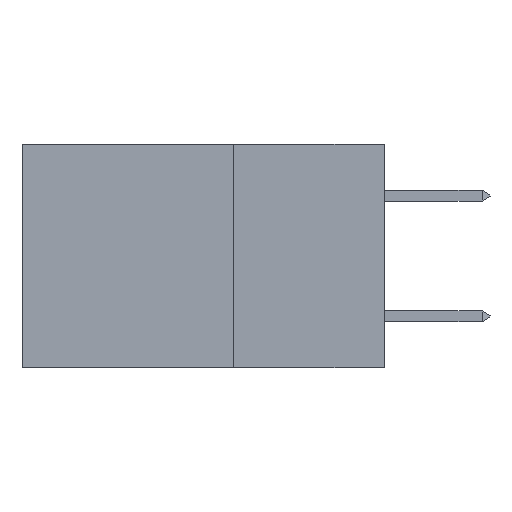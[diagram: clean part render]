
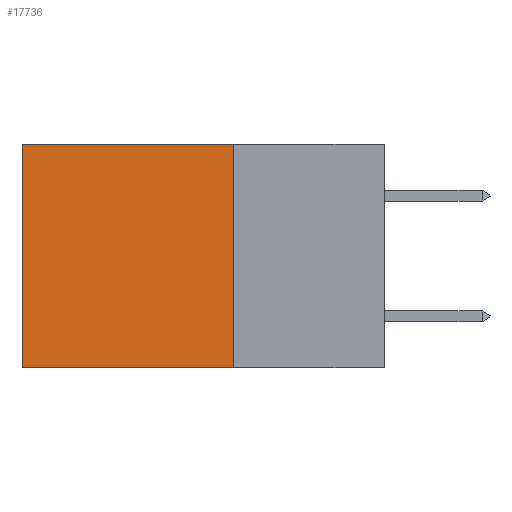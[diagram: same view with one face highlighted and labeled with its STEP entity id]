
A CAD part, left-side view. The second image highlights one B-rep face of the part: STEP entity #17736.
In plain terms, the highlighted planar face has unit normal (-1, 0, 0).
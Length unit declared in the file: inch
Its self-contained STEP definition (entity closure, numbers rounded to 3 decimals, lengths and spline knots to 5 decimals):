
#1192 = CARTESIAN_POINT ( 'NONE',  ( 0.2875, 0.25, 0. ) ) ;
#1269 = DIRECTION ( 'NONE',  ( 0., 0., -1. ) ) ;
#1307 = CARTESIAN_POINT ( 'NONE',  ( 0.2875, 0.25, 0. ) ) ;
#2939 = CARTESIAN_POINT ( 'NONE',  ( 0.2875, 0.6, 0. ) ) ;
#3138 = EDGE_CURVE ( 'NONE', #11681, #18359, #30716, .T. ) ;
#4336 = PLANE ( 'NONE',  #13018 ) ;
#5153 = LINE ( 'NONE', #30262, #12876 ) ;
#6376 = ORIENTED_EDGE ( 'NONE', *, *, #12893, .F. ) ;
#7089 = FACE_OUTER_BOUND ( 'NONE', #10505, .T. ) ;
#8342 = ORIENTED_EDGE ( 'NONE', *, *, #3138, .T. ) ;
#10505 = EDGE_LOOP ( 'NONE', ( #25485, #22693, #6376, #8342 ) ) ;
#11681 = VERTEX_POINT ( 'NONE', #31627 ) ;
#12072 = VERTEX_POINT ( 'NONE', #29418 ) ;
#12851 = LINE ( 'NONE', #24617, #19726 ) ;
#12876 = VECTOR ( 'NONE', #17858, 39.37008 ) ;
#12893 = EDGE_CURVE ( 'NONE', #11681, #12072, #31317, .T. ) ;
#13018 = AXIS2_PLACEMENT_3D ( 'NONE', #24222, #26980, #1269 ) ;
#15668 = DIRECTION ( 'NONE',  ( 0., 0., -1. ) ) ;
#17736 = ADVANCED_FACE ( 'NONE', ( #7089 ), #4336, .F. ) ;
#17858 = DIRECTION ( 'NONE',  ( 0., 1., 0. ) ) ;
#18359 = VERTEX_POINT ( 'NONE', #2939 ) ;
#18795 = EDGE_CURVE ( 'NONE', #18359, #22920, #12851, .T. ) ;
#19726 = VECTOR ( 'NONE', #22470, 39.37008 ) ;
#22390 = EDGE_CURVE ( 'NONE', #12072, #22920, #5153, .T. ) ;
#22470 = DIRECTION ( 'NONE',  ( 0., 0., -1. ) ) ;
#22693 = ORIENTED_EDGE ( 'NONE', *, *, #22390, .F. ) ;
#22920 = VERTEX_POINT ( 'NONE', #31034 ) ;
#22956 = VECTOR ( 'NONE', #28579, 39.37008 ) ;
#23727 = VECTOR ( 'NONE', #15668, 39.37008 ) ;
#24222 = CARTESIAN_POINT ( 'NONE',  ( 0.2875, 0.25, 0. ) ) ;
#24617 = CARTESIAN_POINT ( 'NONE',  ( 0.2875, 0.6, 0. ) ) ;
#25485 = ORIENTED_EDGE ( 'NONE', *, *, #18795, .T. ) ;
#26980 = DIRECTION ( 'NONE',  ( 1., 0., 0. ) ) ;
#28579 = DIRECTION ( 'NONE',  ( 0., 1., 0. ) ) ;
#29418 = CARTESIAN_POINT ( 'NONE',  ( 0.2875, 0.25, -0.37 ) ) ;
#30262 = CARTESIAN_POINT ( 'NONE',  ( 0.2875, 0.25, -0.37 ) ) ;
#30716 = LINE ( 'NONE', #1192, #22956 ) ;
#31034 = CARTESIAN_POINT ( 'NONE',  ( 0.2875, 0.6, -0.37 ) ) ;
#31317 = LINE ( 'NONE', #1307, #23727 ) ;
#31627 = CARTESIAN_POINT ( 'NONE',  ( 0.2875, 0.25, 0. ) ) ;
